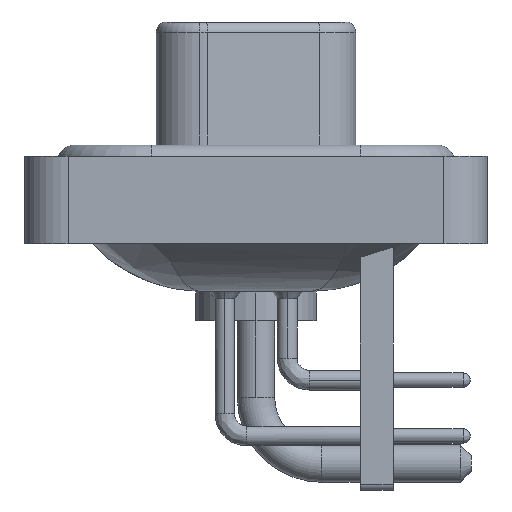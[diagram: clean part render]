
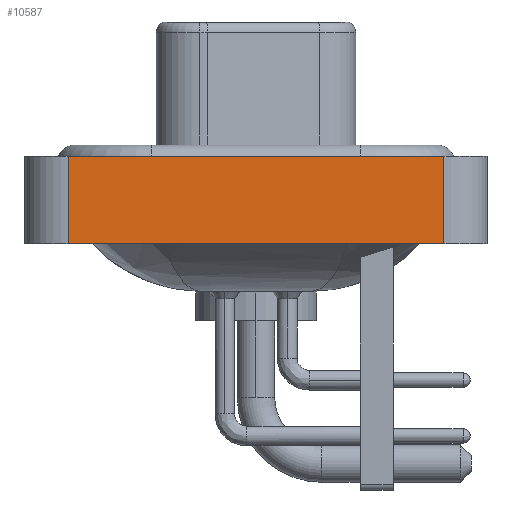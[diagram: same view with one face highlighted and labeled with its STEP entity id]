
A CAD part, left-side view. The second image highlights one B-rep face of the part: STEP entity #10587.
In plain terms, the highlighted planar face has unit normal (-1, 0, 0).
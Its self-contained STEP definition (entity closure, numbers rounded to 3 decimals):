
#180 = AXIS2_PLACEMENT_3D ( 'NONE', #13418, #650, #15201 ) ;
#389 = DIRECTION ( 'NONE',  ( 0., -1., 0. ) ) ;
#650 = DIRECTION ( 'NONE',  ( -1., 0., 0. ) ) ;
#1249 = VECTOR ( 'NONE', #389, 1000. ) ;
#1745 = EDGE_CURVE ( 'NONE', #18126, #13641, #3886, .T. ) ;
#2539 = DIRECTION ( 'NONE',  ( 0., 0., 1. ) ) ;
#2785 = LINE ( 'NONE', #11851, #4885 ) ;
#3886 = LINE ( 'NONE', #9587, #22640 ) ;
#4885 = VECTOR ( 'NONE', #5054, 1000. ) ;
#5054 = DIRECTION ( 'NONE',  ( 0., 0., 1. ) ) ;
#5467 = DIRECTION ( 'NONE',  ( 0., -1., 0. ) ) ;
#5604 = CARTESIAN_POINT ( 'NONE',  ( -7.25, -8.55, -3.6 ) ) ;
#6012 = EDGE_LOOP ( 'NONE', ( #15128, #11738, #6913, #8743 ) ) ;
#6913 = ORIENTED_EDGE ( 'NONE', *, *, #17112, .F. ) ;
#7796 = CARTESIAN_POINT ( 'NONE',  ( -7.25, 8.55, 0.4 ) ) ;
#8743 = ORIENTED_EDGE ( 'NONE', *, *, #20104, .T. ) ;
#8908 = VERTEX_POINT ( 'NONE', #7796 ) ;
#9140 = VECTOR ( 'NONE', #5467, 1000. ) ;
#9445 = CARTESIAN_POINT ( 'NONE',  ( -7.25, -8.55, -3.6 ) ) ;
#9587 = CARTESIAN_POINT ( 'NONE',  ( -7.25, -8.55, -3.6 ) ) ;
#9913 = CARTESIAN_POINT ( 'NONE',  ( -7.25, -8.55, 0.4 ) ) ;
#10587 = ADVANCED_FACE ( 'NONE', ( #22636 ), #19295, .T. ) ;
#11101 = CARTESIAN_POINT ( 'NONE',  ( -7.25, 8.55, -3.6 ) ) ;
#11183 = CARTESIAN_POINT ( 'NONE',  ( -7.25, -8.55, 0.4 ) ) ;
#11238 = LINE ( 'NONE', #9445, #1249 ) ;
#11738 = ORIENTED_EDGE ( 'NONE', *, *, #15126, .F. ) ;
#11851 = CARTESIAN_POINT ( 'NONE',  ( -7.25, 8.55, -3.6 ) ) ;
#12695 = VERTEX_POINT ( 'NONE', #11101 ) ;
#13418 = CARTESIAN_POINT ( 'NONE',  ( -7.25, -8.55, -3.6 ) ) ;
#13641 = VERTEX_POINT ( 'NONE', #9913 ) ;
#15126 = EDGE_CURVE ( 'NONE', #8908, #13641, #21741, .T. ) ;
#15128 = ORIENTED_EDGE ( 'NONE', *, *, #1745, .T. ) ;
#15201 = DIRECTION ( 'NONE',  ( 0., 0., 1. ) ) ;
#17112 = EDGE_CURVE ( 'NONE', #12695, #8908, #2785, .T. ) ;
#18126 = VERTEX_POINT ( 'NONE', #5604 ) ;
#19295 = PLANE ( 'NONE',  #180 ) ;
#20104 = EDGE_CURVE ( 'NONE', #12695, #18126, #11238, .T. ) ;
#21741 = LINE ( 'NONE', #11183, #9140 ) ;
#22636 = FACE_OUTER_BOUND ( 'NONE', #6012, .T. ) ;
#22640 = VECTOR ( 'NONE', #2539, 1000. ) ;
